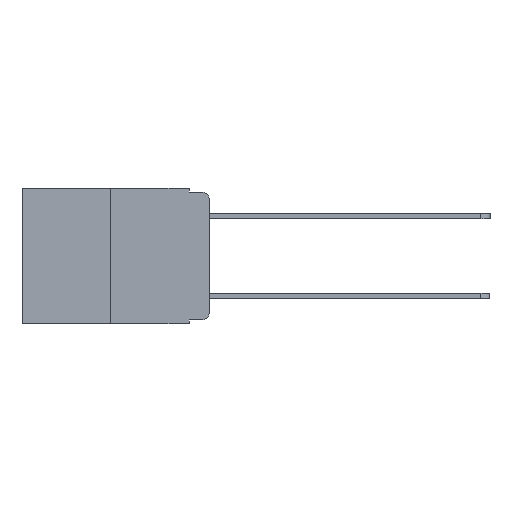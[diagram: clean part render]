
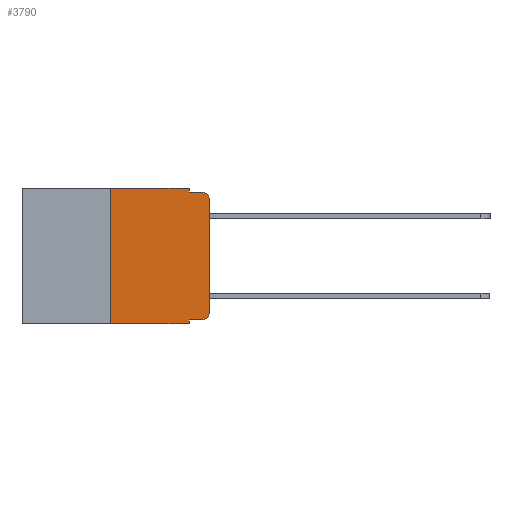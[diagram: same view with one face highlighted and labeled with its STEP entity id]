
A CAD part, left-side view. The second image highlights one B-rep face of the part: STEP entity #3790.
In plain terms, the highlighted planar face has unit normal (-1, 0, 0).
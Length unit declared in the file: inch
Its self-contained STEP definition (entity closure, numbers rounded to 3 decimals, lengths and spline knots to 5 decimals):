
#333 = DIRECTION ( 'NONE',  ( 0., 0., -1. ) ) ;
#464 = EDGE_CURVE ( 'NONE', #3966, #10157, #9254, .T. ) ;
#688 = VECTOR ( 'NONE', #1513, 39.37008 ) ;
#796 = CARTESIAN_POINT ( 'NONE',  ( 0., 0.02, -0.313 ) ) ;
#869 = VERTEX_POINT ( 'NONE', #1648 ) ;
#982 = CARTESIAN_POINT ( 'NONE',  ( 0., 0., -0.313 ) ) ;
#1163 = VERTEX_POINT ( 'NONE', #3953 ) ;
#1169 = DIRECTION ( 'NONE',  ( 0., -1., 0. ) ) ;
#1309 = ORIENTED_EDGE ( 'NONE', *, *, #3486, .F. ) ;
#1360 = VERTEX_POINT ( 'NONE', #9130 ) ;
#1465 = CARTESIAN_POINT ( 'NONE',  ( 0., 0.473, 0. ) ) ;
#1513 = DIRECTION ( 'NONE',  ( 0., -1., 0. ) ) ;
#1648 = CARTESIAN_POINT ( 'NONE',  ( 0., 0.051, -0.333 ) ) ;
#1746 = ORIENTED_EDGE ( 'NONE', *, *, #3721, .F. ) ;
#1906 = EDGE_CURVE ( 'NONE', #10157, #2092, #9581, .T. ) ;
#1978 = CARTESIAN_POINT ( 'NONE',  ( 0., 0., -0.03 ) ) ;
#2092 = VERTEX_POINT ( 'NONE', #1978 ) ;
#2284 = DIRECTION ( 'NONE',  ( 0., 0., -1. ) ) ;
#2402 = DIRECTION ( 'NONE',  ( 0., 0., -1. ) ) ;
#2479 = VERTEX_POINT ( 'NONE', #8128 ) ;
#2588 = CARTESIAN_POINT ( 'NONE',  ( 0., 0.051, -0.343 ) ) ;
#2822 = CARTESIAN_POINT ( 'NONE',  ( 0., 0.473, -0.343 ) ) ;
#2959 = ORIENTED_EDGE ( 'NONE', *, *, #10573, .F. ) ;
#3091 = AXIS2_PLACEMENT_3D ( 'NONE', #10941, #5925, #333 ) ;
#3124 = ORIENTED_EDGE ( 'NONE', *, *, #11088, .F. ) ;
#3206 = EDGE_CURVE ( 'NONE', #1360, #4754, #4756, .T. ) ;
#3240 = VECTOR ( 'NONE', #10366, 39.37008 ) ;
#3355 = ORIENTED_EDGE ( 'NONE', *, *, #3206, .T. ) ;
#3430 = CARTESIAN_POINT ( 'NONE',  ( 0., 0.051, -0.01 ) ) ;
#3467 = DIRECTION ( 'NONE',  ( 0., -1., 0. ) ) ;
#3486 = EDGE_CURVE ( 'NONE', #1360, #2479, #9503, .T. ) ;
#3721 = EDGE_CURVE ( 'NONE', #5717, #6555, #4536, .T. ) ;
#3790 = ADVANCED_FACE ( 'NONE', ( #6053 ), #6060, .F. ) ;
#3953 = CARTESIAN_POINT ( 'NONE',  ( 0., 0.02, -0.01 ) ) ;
#3966 = VERTEX_POINT ( 'NONE', #8102 ) ;
#4011 = CIRCLE ( 'NONE', #3091, 0.02 ) ;
#4536 = LINE ( 'NONE', #7710, #11295 ) ;
#4754 = VERTEX_POINT ( 'NONE', #2588 ) ;
#4756 = LINE ( 'NONE', #2822, #688 ) ;
#4954 = CARTESIAN_POINT ( 'NONE',  ( 0., 0.051, -0.333 ) ) ;
#5622 = AXIS2_PLACEMENT_3D ( 'NONE', #1465, #7813, #2402 ) ;
#5717 = VERTEX_POINT ( 'NONE', #9180 ) ;
#5722 = EDGE_CURVE ( 'NONE', #869, #3966, #8428, .T. ) ;
#5880 = VECTOR ( 'NONE', #1169, 39.37008 ) ;
#5925 = DIRECTION ( 'NONE',  ( -1., 0., 0. ) ) ;
#5943 = LINE ( 'NONE', #9542, #3240 ) ;
#6053 = FACE_OUTER_BOUND ( 'NONE', #9225, .T. ) ;
#6060 = PLANE ( 'NONE',  #5622 ) ;
#6064 = VECTOR ( 'NONE', #10739, 39.37008 ) ;
#6555 = VERTEX_POINT ( 'NONE', #3430 ) ;
#6860 = VECTOR ( 'NONE', #11013, 39.37008 ) ;
#7038 = EDGE_CURVE ( 'NONE', #2092, #1163, #4011, .T. ) ;
#7041 = ORIENTED_EDGE ( 'NONE', *, *, #464, .T. ) ;
#7155 = ORIENTED_EDGE ( 'NONE', *, *, #9345, .F. ) ;
#7710 = CARTESIAN_POINT ( 'NONE',  ( 0., 0.051, 0. ) ) ;
#7813 = DIRECTION ( 'NONE',  ( 1., 0., 0. ) ) ;
#8102 = CARTESIAN_POINT ( 'NONE',  ( 0., 0.02, -0.333 ) ) ;
#8128 = CARTESIAN_POINT ( 'NONE',  ( 0., 0.25, 0. ) ) ;
#8245 = ORIENTED_EDGE ( 'NONE', *, *, #7038, .T. ) ;
#8297 = DIRECTION ( 'NONE',  ( 0., 0., -1. ) ) ;
#8428 = LINE ( 'NONE', #4954, #5880 ) ;
#8913 = CARTESIAN_POINT ( 'NONE',  ( 0., 0., 0. ) ) ;
#8998 = AXIS2_PLACEMENT_3D ( 'NONE', #796, #9166, #8297 ) ;
#9130 = CARTESIAN_POINT ( 'NONE',  ( 0., 0.25, -0.343 ) ) ;
#9133 = CARTESIAN_POINT ( 'NONE',  ( 0., 0.473, 0. ) ) ;
#9136 = LINE ( 'NONE', #10381, #11062 ) ;
#9166 = DIRECTION ( 'NONE',  ( -1., 0., 0. ) ) ;
#9180 = CARTESIAN_POINT ( 'NONE',  ( 0., 0.051, 0. ) ) ;
#9225 = EDGE_LOOP ( 'NONE', ( #11467, #8245, #2959, #1746, #3124, #1309, #3355, #7155, #9496, #7041 ) ) ;
#9254 = CIRCLE ( 'NONE', #8998, 0.02 ) ;
#9345 = EDGE_CURVE ( 'NONE', #869, #4754, #5943, .T. ) ;
#9496 = ORIENTED_EDGE ( 'NONE', *, *, #5722, .T. ) ;
#9503 = LINE ( 'NONE', #9803, #11428 ) ;
#9542 = CARTESIAN_POINT ( 'NONE',  ( 0., 0.051, 0. ) ) ;
#9581 = LINE ( 'NONE', #8913, #6860 ) ;
#9803 = CARTESIAN_POINT ( 'NONE',  ( 0., 0.25, 0. ) ) ;
#10157 = VERTEX_POINT ( 'NONE', #982 ) ;
#10366 = DIRECTION ( 'NONE',  ( 0., 0., -1. ) ) ;
#10381 = CARTESIAN_POINT ( 'NONE',  ( 0., 0.051, -0.01 ) ) ;
#10573 = EDGE_CURVE ( 'NONE', #6555, #1163, #9136, .T. ) ;
#10621 = DIRECTION ( 'NONE',  ( 0., 0., 1. ) ) ;
#10739 = DIRECTION ( 'NONE',  ( 0., -1., 0. ) ) ;
#10785 = LINE ( 'NONE', #9133, #6064 ) ;
#10941 = CARTESIAN_POINT ( 'NONE',  ( 0., 0.02, -0.03 ) ) ;
#11013 = DIRECTION ( 'NONE',  ( 0., 0., 1. ) ) ;
#11062 = VECTOR ( 'NONE', #3467, 39.37008 ) ;
#11088 = EDGE_CURVE ( 'NONE', #2479, #5717, #10785, .T. ) ;
#11295 = VECTOR ( 'NONE', #2284, 39.37008 ) ;
#11428 = VECTOR ( 'NONE', #10621, 39.37008 ) ;
#11467 = ORIENTED_EDGE ( 'NONE', *, *, #1906, .T. ) ;
